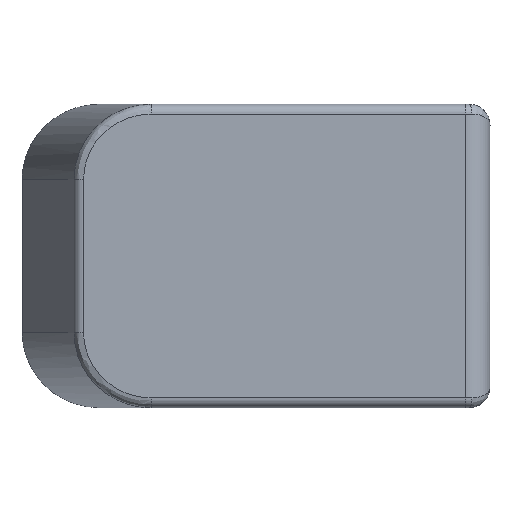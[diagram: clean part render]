
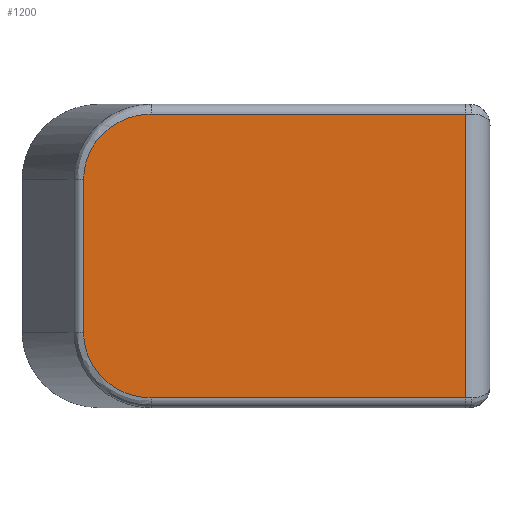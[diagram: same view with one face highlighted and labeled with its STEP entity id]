
A CAD part, front view. The second image highlights one B-rep face of the part: STEP entity #1200.
In plain terms, the highlighted planar face has unit normal (0, -1, 0).
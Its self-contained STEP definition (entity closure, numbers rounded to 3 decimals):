
#80=FACE_OUTER_BOUND('',#152,.T.);
#152=EDGE_LOOP('',(#937,#938,#939,#940,#941,#942));
#217=ELLIPSE('',#1321,6.854,6.62);
#218=ELLIPSE('',#1322,6.854,6.62);
#291=LINE('',#2011,#405);
#323=LINE('',#2095,#437);
#326=LINE('',#2105,#440);
#327=LINE('',#2109,#441);
#405=VECTOR('',#1488,10.);
#437=VECTOR('',#1558,10.);
#440=VECTOR('',#1571,10.);
#441=VECTOR('',#1574,10.);
#524=VERTEX_POINT('',#1871);
#527=VERTEX_POINT('',#1911);
#567=VERTEX_POINT('',#2094);
#569=VERTEX_POINT('',#2104);
#570=VERTEX_POINT('',#2106);
#571=VERTEX_POINT('',#2108);
#659=EDGE_CURVE('',#524,#527,#291,.T.);
#702=EDGE_CURVE('',#527,#567,#323,.T.);
#707=EDGE_CURVE('',#569,#524,#326,.T.);
#708=EDGE_CURVE('',#570,#569,#217,.T.);
#709=EDGE_CURVE('',#571,#570,#327,.T.);
#710=EDGE_CURVE('',#567,#571,#218,.T.);
#937=ORIENTED_EDGE('',*,*,#659,.F.);
#938=ORIENTED_EDGE('',*,*,#707,.F.);
#939=ORIENTED_EDGE('',*,*,#708,.F.);
#940=ORIENTED_EDGE('',*,*,#709,.F.);
#941=ORIENTED_EDGE('',*,*,#710,.F.);
#942=ORIENTED_EDGE('',*,*,#702,.F.);
#1151=PLANE('',#1320);
#1200=ADVANCED_FACE('',(#80),#1151,.F.);
#1320=AXIS2_PLACEMENT_3D('',#2103,#1569,#1570);
#1321=AXIS2_PLACEMENT_3D('',#2107,#1572,#1573);
#1322=AXIS2_PLACEMENT_3D('',#2110,#1575,#1576);
#1488=DIRECTION('',(0.,0.,-1.));
#1558=DIRECTION('',(-1.,0.,0.));
#1569=DIRECTION('center_axis',(0.,1.,0.));
#1570=DIRECTION('ref_axis',(0.,0.,1.));
#1571=DIRECTION('',(1.,0.,0.));
#1572=DIRECTION('center_axis',(0.,1.,0.));
#1573=DIRECTION('ref_axis',(-1.,0.,0.));
#1574=DIRECTION('',(0.,0.,1.));
#1575=DIRECTION('center_axis',(0.,1.,0.));
#1576=DIRECTION('ref_axis',(-1.,0.,0.));
#1871=CARTESIAN_POINT('',(43.285,-15.,0.));
#1911=CARTESIAN_POINT('',(43.285,-15.,-28.778));
#2011=CARTESIAN_POINT('',(43.285,-15.,-7.195));
#2094=CARTESIAN_POINT('',(11.413,-15.,-28.778));
#2095=CARTESIAN_POINT('',(29.489,-15.,-28.778));
#2103=CARTESIAN_POINT('Origin',(19.66,-15.,-14.389));
#2104=CARTESIAN_POINT('',(11.413,-15.,0.));
#2105=CARTESIAN_POINT('',(9.83,-15.,0.));
#2106=CARTESIAN_POINT('',(4.559,-15.,-6.62));
#2107=CARTESIAN_POINT('Origin',(11.413,-15.,-6.62));
#2108=CARTESIAN_POINT('',(4.559,-15.,-22.158));
#2109=CARTESIAN_POINT('',(4.559,-15.,-21.584));
#2110=CARTESIAN_POINT('Origin',(11.413,-15.,-22.158));
